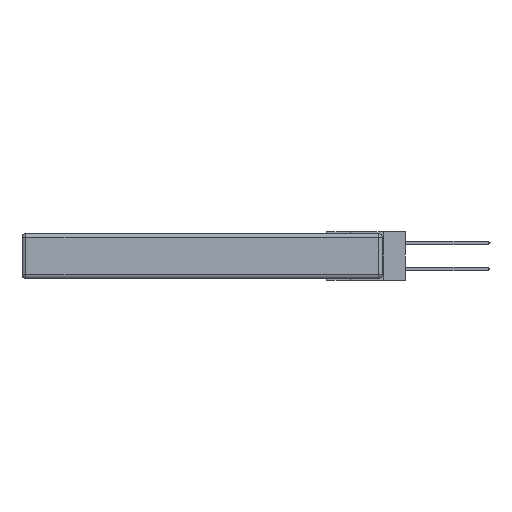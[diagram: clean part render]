
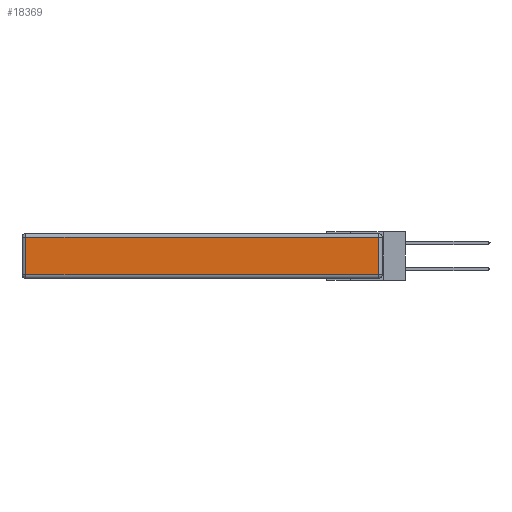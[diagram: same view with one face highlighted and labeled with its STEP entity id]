
A CAD part, left-side view. The second image highlights one B-rep face of the part: STEP entity #18369.
In plain terms, the highlighted planar face has unit normal (-1, 0, 0).
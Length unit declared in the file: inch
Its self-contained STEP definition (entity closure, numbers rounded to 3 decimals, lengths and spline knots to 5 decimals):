
#196 = ORIENTED_EDGE ( 'NONE', *, *, #14689, .T. ) ;
#985 = DIRECTION ( 'NONE',  ( 0., 0., -1. ) ) ;
#1063 = CARTESIAN_POINT ( 'NONE',  ( 0., 2.72, -0.343 ) ) ;
#1095 = VERTEX_POINT ( 'NONE', #21893 ) ;
#2484 = VECTOR ( 'NONE', #2892, 39.37008 ) ;
#2892 = DIRECTION ( 'NONE',  ( 0., -1., 0. ) ) ;
#3671 = DIRECTION ( 'NONE',  ( 0., 0., 1. ) ) ;
#4017 = CARTESIAN_POINT ( 'NONE',  ( 0., 0.03, -0.03 ) ) ;
#4341 = EDGE_LOOP ( 'NONE', ( #19322, #12588, #196, #18948 ) ) ;
#4757 = CARTESIAN_POINT ( 'NONE',  ( 0., 0., -0.313 ) ) ;
#5200 = LINE ( 'NONE', #6777, #15311 ) ;
#5218 = FACE_OUTER_BOUND ( 'NONE', #4341, .T. ) ;
#5422 = EDGE_CURVE ( 'NONE', #21933, #7157, #13450, .T. ) ;
#5697 = CARTESIAN_POINT ( 'NONE',  ( 0., 0.03, -0.343 ) ) ;
#6777 = CARTESIAN_POINT ( 'NONE',  ( 0., 2.75, -0.03 ) ) ;
#7157 = VERTEX_POINT ( 'NONE', #4017 ) ;
#7663 = EDGE_CURVE ( 'NONE', #20451, #21933, #10613, .T. ) ;
#10454 = AXIS2_PLACEMENT_3D ( 'NONE', #14093, #19562, #3671 ) ;
#10613 = LINE ( 'NONE', #4757, #2484 ) ;
#11142 = CARTESIAN_POINT ( 'NONE',  ( 0., 0.03, -0.313 ) ) ;
#12588 = ORIENTED_EDGE ( 'NONE', *, *, #5422, .T. ) ;
#12593 = VECTOR ( 'NONE', #12701, 39.37008 ) ;
#12701 = DIRECTION ( 'NONE',  ( 0., 0., 1. ) ) ;
#13450 = LINE ( 'NONE', #5697, #12593 ) ;
#14093 = CARTESIAN_POINT ( 'NONE',  ( 0., 0., -0.343 ) ) ;
#14689 = EDGE_CURVE ( 'NONE', #7157, #1095, #5200, .T. ) ;
#15311 = VECTOR ( 'NONE', #20615, 39.37008 ) ;
#16081 = PLANE ( 'NONE',  #10454 ) ;
#16315 = CARTESIAN_POINT ( 'NONE',  ( 0., 2.72, -0.313 ) ) ;
#16778 = VECTOR ( 'NONE', #985, 39.37008 ) ;
#18369 = ADVANCED_FACE ( 'NONE', ( #5218 ), #16081, .T. ) ;
#18948 = ORIENTED_EDGE ( 'NONE', *, *, #19242, .T. ) ;
#19242 = EDGE_CURVE ( 'NONE', #1095, #20451, #19479, .T. ) ;
#19322 = ORIENTED_EDGE ( 'NONE', *, *, #7663, .T. ) ;
#19479 = LINE ( 'NONE', #1063, #16778 ) ;
#19562 = DIRECTION ( 'NONE',  ( -1., 0., 0. ) ) ;
#20451 = VERTEX_POINT ( 'NONE', #16315 ) ;
#20615 = DIRECTION ( 'NONE',  ( 0., 1., 0. ) ) ;
#21893 = CARTESIAN_POINT ( 'NONE',  ( 0., 2.72, -0.03 ) ) ;
#21933 = VERTEX_POINT ( 'NONE', #11142 ) ;
